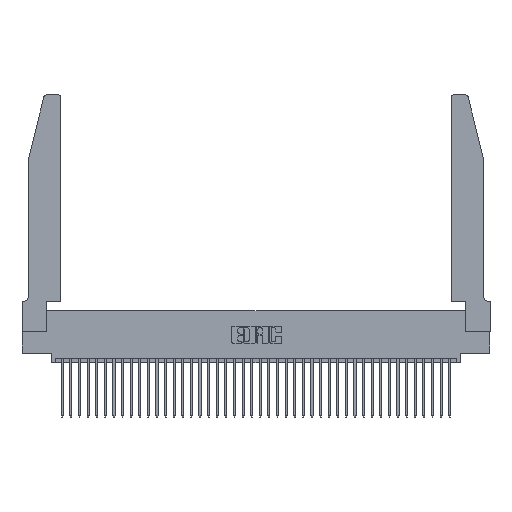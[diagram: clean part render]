
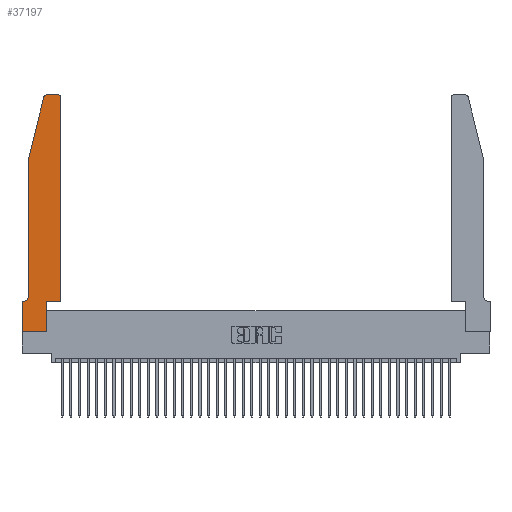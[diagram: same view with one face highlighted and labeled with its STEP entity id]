
A CAD part, top view. The second image highlights one B-rep face of the part: STEP entity #37197.
In plain terms, the highlighted planar face has unit normal (0, 0, 1).
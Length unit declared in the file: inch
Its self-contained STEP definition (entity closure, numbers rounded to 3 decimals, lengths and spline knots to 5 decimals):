
#170 = CARTESIAN_POINT ( 'NONE',  ( 0.2605, 2.75, 0.37 ) ) ;
#910 = VERTEX_POINT ( 'NONE', #27497 ) ;
#946 = CARTESIAN_POINT ( 'NONE',  ( 0.0055, 0.42, 0.37 ) ) ;
#1228 = CARTESIAN_POINT ( 'NONE',  ( 0., 0.35, 0.37 ) ) ;
#1818 = VERTEX_POINT ( 'NONE', #21199 ) ;
#2363 = CARTESIAN_POINT ( 'NONE',  ( 0.4205, 2.75, 0.37 ) ) ;
#2546 = CARTESIAN_POINT ( 'NONE',  ( 0.284, 2.72, 0.37 ) ) ;
#2632 = VECTOR ( 'NONE', #21362, 39.37008 ) ;
#2909 = ORIENTED_EDGE ( 'NONE', *, *, #38390, .T. ) ;
#3045 = EDGE_CURVE ( 'NONE', #25806, #1818, #37802, .T. ) ;
#4385 = CARTESIAN_POINT ( 'NONE',  ( 0.4205, 2.72, 0.37 ) ) ;
#5281 = CIRCLE ( 'NONE', #14048, 0.03 ) ;
#5692 = EDGE_CURVE ( 'NONE', #910, #13036, #37344, .T. ) ;
#6228 = DIRECTION ( 'NONE',  ( 0., 1., 0. ) ) ;
#6301 = ORIENTED_EDGE ( 'NONE', *, *, #30682, .T. ) ;
#6777 = DIRECTION ( 'NONE',  ( 1., 0., 0. ) ) ;
#7750 = AXIS2_PLACEMENT_3D ( 'NONE', #27051, #20742, #27309 ) ;
#8566 = VERTEX_POINT ( 'NONE', #16384 ) ;
#9089 = CARTESIAN_POINT ( 'NONE',  ( 0.2865, 0.35, 0.37 ) ) ;
#9541 = CARTESIAN_POINT ( 'NONE',  ( 0., 0., 0.37 ) ) ;
#10530 = AXIS2_PLACEMENT_3D ( 'NONE', #2546, #18087, #14771 ) ;
#11253 = PLANE ( 'NONE',  #7750 ) ;
#11637 = CARTESIAN_POINT ( 'NONE',  ( 0.2865, 0., 0.37 ) ) ;
#12022 = CARTESIAN_POINT ( 'NONE',  ( 0.4505, 0.35, 0.37 ) ) ;
#12295 = VECTOR ( 'NONE', #24949, 39.37008 ) ;
#13036 = VERTEX_POINT ( 'NONE', #33036 ) ;
#13258 = LINE ( 'NONE', #17131, #15729 ) ;
#13267 = VECTOR ( 'NONE', #15242, 39.37008 ) ;
#13577 = LINE ( 'NONE', #39781, #33263 ) ;
#13579 = VERTEX_POINT ( 'NONE', #1228 ) ;
#14048 = AXIS2_PLACEMENT_3D ( 'NONE', #4385, #26550, #26289 ) ;
#14162 = EDGE_CURVE ( 'NONE', #16289, #27224, #35894, .T. ) ;
#14330 = EDGE_CURVE ( 'NONE', #8566, #16860, #13258, .T. ) ;
#14771 = DIRECTION ( 'NONE',  ( 1., 0., 0. ) ) ;
#14785 = AXIS2_PLACEMENT_3D ( 'NONE', #946, #28048, #20883 ) ;
#15242 = DIRECTION ( 'NONE',  ( -1., 0., 0. ) ) ;
#15729 = VECTOR ( 'NONE', #39077, 39.37008 ) ;
#15868 = LINE ( 'NONE', #30290, #38958 ) ;
#15974 = ORIENTED_EDGE ( 'NONE', *, *, #36363, .T. ) ;
#16289 = VERTEX_POINT ( 'NONE', #40202 ) ;
#16313 = EDGE_CURVE ( 'NONE', #13579, #20335, #13577, .T. ) ;
#16384 = CARTESIAN_POINT ( 'NONE',  ( 0.25487, 2.72718, 0.37 ) ) ;
#16600 = ORIENTED_EDGE ( 'NONE', *, *, #16313, .T. ) ;
#16860 = VERTEX_POINT ( 'NONE', #21904 ) ;
#17131 = CARTESIAN_POINT ( 'NONE',  ( 0.0755, 2., 0.37 ) ) ;
#17361 = ORIENTED_EDGE ( 'NONE', *, *, #14162, .T. ) ;
#18087 = DIRECTION ( 'NONE',  ( 0., 0., 1. ) ) ;
#18411 = FACE_OUTER_BOUND ( 'NONE', #39199, .T. ) ;
#20335 = VERTEX_POINT ( 'NONE', #9541 ) ;
#20742 = DIRECTION ( 'NONE',  ( 0., 0., 1. ) ) ;
#20883 = DIRECTION ( 'NONE',  ( -1., 0., 0. ) ) ;
#21199 = CARTESIAN_POINT ( 'NONE',  ( 0.284, 2.75, 0.37 ) ) ;
#21279 = ORIENTED_EDGE ( 'NONE', *, *, #3045, .T. ) ;
#21362 = DIRECTION ( 'NONE',  ( 0., -1., 0. ) ) ;
#21452 = VECTOR ( 'NONE', #6777, 39.37008 ) ;
#21904 = CARTESIAN_POINT ( 'NONE',  ( 0.0755, 2., 0.37 ) ) ;
#22721 = VERTEX_POINT ( 'NONE', #35086 ) ;
#23391 = LINE ( 'NONE', #37129, #21452 ) ;
#23719 = ORIENTED_EDGE ( 'NONE', *, *, #26011, .T. ) ;
#24366 = CARTESIAN_POINT ( 'NONE',  ( 0.0755, 2., 0.37 ) ) ;
#24949 = DIRECTION ( 'NONE',  ( 1., 0., 0. ) ) ;
#25643 = ORIENTED_EDGE ( 'NONE', *, *, #33449, .T. ) ;
#25656 = LINE ( 'NONE', #12022, #27640 ) ;
#25806 = VERTEX_POINT ( 'NONE', #2363 ) ;
#26011 = EDGE_CURVE ( 'NONE', #20335, #29175, #23391, .T. ) ;
#26289 = DIRECTION ( 'NONE',  ( 1., 0., 0. ) ) ;
#26550 = DIRECTION ( 'NONE',  ( 0., 0., 1. ) ) ;
#26958 = CARTESIAN_POINT ( 'NONE',  ( 0.0055, 0.35, 0.37 ) ) ;
#27051 = CARTESIAN_POINT ( 'NONE',  ( 0., 0.35, 0.37 ) ) ;
#27224 = VERTEX_POINT ( 'NONE', #26958 ) ;
#27309 = DIRECTION ( 'NONE',  ( 1., 0., 0. ) ) ;
#27497 = CARTESIAN_POINT ( 'NONE',  ( 0.2865, 0.35, 0.37 ) ) ;
#27640 = VECTOR ( 'NONE', #34020, 39.37008 ) ;
#28048 = DIRECTION ( 'NONE',  ( 0., 0., -1. ) ) ;
#29175 = VERTEX_POINT ( 'NONE', #11637 ) ;
#29393 = CIRCLE ( 'NONE', #10530, 0.03 ) ;
#29666 = ORIENTED_EDGE ( 'NONE', *, *, #31086, .T. ) ;
#29755 = ORIENTED_EDGE ( 'NONE', *, *, #33033, .T. ) ;
#29902 = LINE ( 'NONE', #9089, #34325 ) ;
#30290 = CARTESIAN_POINT ( 'NONE',  ( 0.0755, 0.35, 0.37 ) ) ;
#30329 = ORIENTED_EDGE ( 'NONE', *, *, #5692, .T. ) ;
#30682 = EDGE_CURVE ( 'NONE', #29175, #910, #29902, .T. ) ;
#31086 = EDGE_CURVE ( 'NONE', #1818, #8566, #29393, .T. ) ;
#33033 = EDGE_CURVE ( 'NONE', #13036, #22721, #25656, .T. ) ;
#33036 = CARTESIAN_POINT ( 'NONE',  ( 0.4505, 0.35, 0.37 ) ) ;
#33263 = VECTOR ( 'NONE', #40072, 39.37008 ) ;
#33449 = EDGE_CURVE ( 'NONE', #16860, #16289, #37870, .T. ) ;
#33580 = ORIENTED_EDGE ( 'NONE', *, *, #14330, .T. ) ;
#34020 = DIRECTION ( 'NONE',  ( 0., 1., 0. ) ) ;
#34325 = VECTOR ( 'NONE', #6228, 39.37008 ) ;
#35086 = CARTESIAN_POINT ( 'NONE',  ( 0.4505, 2.72, 0.37 ) ) ;
#35894 = CIRCLE ( 'NONE', #14785, 0.07 ) ;
#36363 = EDGE_CURVE ( 'NONE', #22721, #25806, #5281, .T. ) ;
#36875 = DIRECTION ( 'NONE',  ( -1., 0., 0. ) ) ;
#37129 = CARTESIAN_POINT ( 'NONE',  ( 0., 0., 0.37 ) ) ;
#37197 = ADVANCED_FACE ( 'NONE', ( #18411 ), #11253, .T. ) ;
#37344 = LINE ( 'NONE', #39229, #12295 ) ;
#37802 = LINE ( 'NONE', #170, #13267 ) ;
#37870 = LINE ( 'NONE', #24366, #2632 ) ;
#38390 = EDGE_CURVE ( 'NONE', #27224, #13579, #15868, .T. ) ;
#38958 = VECTOR ( 'NONE', #36875, 39.37008 ) ;
#39077 = DIRECTION ( 'NONE',  ( -0.239, -0.971, 0. ) ) ;
#39199 = EDGE_LOOP ( 'NONE', ( #21279, #29666, #33580, #25643, #17361, #2909, #16600, #23719, #6301, #30329, #29755, #15974 ) ) ;
#39229 = CARTESIAN_POINT ( 'NONE',  ( 0.4505, 0.35, 0.37 ) ) ;
#39781 = CARTESIAN_POINT ( 'NONE',  ( 0., 0., 0.37 ) ) ;
#40072 = DIRECTION ( 'NONE',  ( 0., -1., 0. ) ) ;
#40202 = CARTESIAN_POINT ( 'NONE',  ( 0.0755, 0.42, 0.37 ) ) ;
